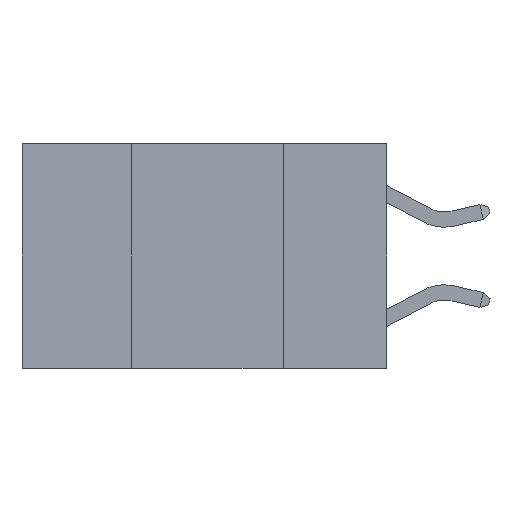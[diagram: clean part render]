
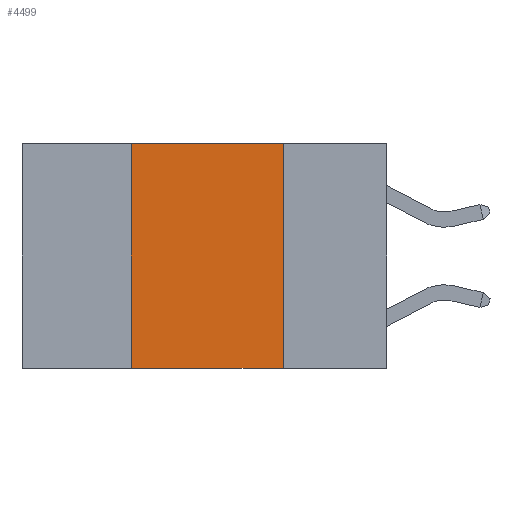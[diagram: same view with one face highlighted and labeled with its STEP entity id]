
A CAD part, left-side view. The second image highlights one B-rep face of the part: STEP entity #4499.
In plain terms, the highlighted planar face has unit normal (-1, 0, 0).
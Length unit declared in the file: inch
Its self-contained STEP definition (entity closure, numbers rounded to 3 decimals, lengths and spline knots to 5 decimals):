
#174 = CARTESIAN_POINT ( 'NONE',  ( 0., 0.17, 0. ) ) ;
#515 = VECTOR ( 'NONE', #9886, 39.37008 ) ;
#613 = EDGE_CURVE ( 'NONE', #6024, #1045, #9648, .T. ) ;
#747 = DIRECTION ( 'NONE',  ( 0., 0., -1. ) ) ;
#818 = LINE ( 'NONE', #11846, #515 ) ;
#900 = CARTESIAN_POINT ( 'NONE',  ( 0., 0.42, 0. ) ) ;
#1010 = CARTESIAN_POINT ( 'NONE',  ( 0., 0.42, -0.37 ) ) ;
#1045 = VERTEX_POINT ( 'NONE', #10262 ) ;
#1106 = CARTESIAN_POINT ( 'NONE',  ( 0., 0.6, 0. ) ) ;
#1314 = EDGE_CURVE ( 'NONE', #4696, #6024, #4363, .T. ) ;
#1481 = AXIS2_PLACEMENT_3D ( 'NONE', #5776, #6757, #747 ) ;
#1879 = CARTESIAN_POINT ( 'NONE',  ( 0., 0.42, 0. ) ) ;
#3252 = DIRECTION ( 'NONE',  ( 0., -1., 0. ) ) ;
#4363 = LINE ( 'NONE', #1879, #6706 ) ;
#4435 = VECTOR ( 'NONE', #3252, 39.37008 ) ;
#4499 = ADVANCED_FACE ( 'NONE', ( #10298 ), #11601, .F. ) ;
#4577 = CARTESIAN_POINT ( 'NONE',  ( 0., 0.17, -0.37 ) ) ;
#4681 = EDGE_CURVE ( 'NONE', #4696, #11276, #818, .T. ) ;
#4696 = VERTEX_POINT ( 'NONE', #1010 ) ;
#4998 = ORIENTED_EDGE ( 'NONE', *, *, #613, .F. ) ;
#5321 = ORIENTED_EDGE ( 'NONE', *, *, #4681, .T. ) ;
#5662 = DIRECTION ( 'NONE',  ( 0., 0., 1. ) ) ;
#5776 = CARTESIAN_POINT ( 'NONE',  ( 0., 0.6, 0. ) ) ;
#6024 = VERTEX_POINT ( 'NONE', #900 ) ;
#6166 = EDGE_LOOP ( 'NONE', ( #7318, #4998, #7611, #5321 ) ) ;
#6194 = DIRECTION ( 'NONE',  ( 0., 0., -1. ) ) ;
#6238 = LINE ( 'NONE', #174, #11707 ) ;
#6706 = VECTOR ( 'NONE', #5662, 39.37008 ) ;
#6757 = DIRECTION ( 'NONE',  ( 1., 0., 0. ) ) ;
#7318 = ORIENTED_EDGE ( 'NONE', *, *, #10187, .F. ) ;
#7611 = ORIENTED_EDGE ( 'NONE', *, *, #1314, .F. ) ;
#9648 = LINE ( 'NONE', #1106, #4435 ) ;
#9886 = DIRECTION ( 'NONE',  ( 0., -1., 0. ) ) ;
#10187 = EDGE_CURVE ( 'NONE', #1045, #11276, #6238, .T. ) ;
#10262 = CARTESIAN_POINT ( 'NONE',  ( 0., 0.17, 0. ) ) ;
#10298 = FACE_OUTER_BOUND ( 'NONE', #6166, .T. ) ;
#11276 = VERTEX_POINT ( 'NONE', #4577 ) ;
#11601 = PLANE ( 'NONE',  #1481 ) ;
#11707 = VECTOR ( 'NONE', #6194, 39.37008 ) ;
#11846 = CARTESIAN_POINT ( 'NONE',  ( 0., 0.6, -0.37 ) ) ;
